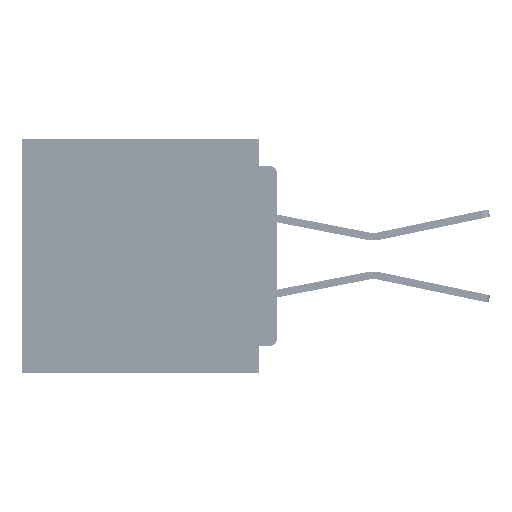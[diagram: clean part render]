
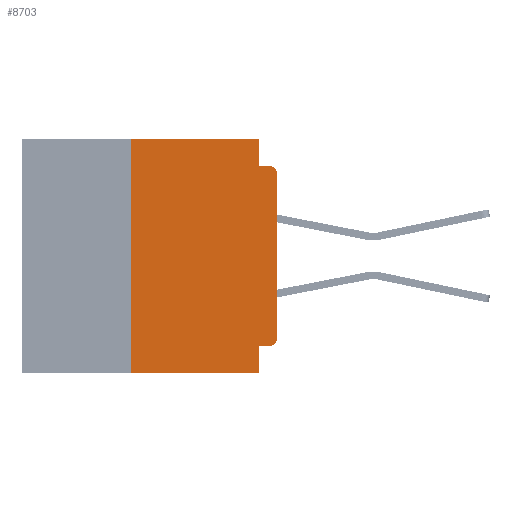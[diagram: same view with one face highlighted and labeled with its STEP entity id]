
A CAD part, left-side view. The second image highlights one B-rep face of the part: STEP entity #8703.
In plain terms, the highlighted planar face has unit normal (-1, 0, 0).
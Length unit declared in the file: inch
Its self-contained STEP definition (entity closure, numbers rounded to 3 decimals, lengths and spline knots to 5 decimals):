
#1179 = ORIENTED_EDGE ( 'NONE', *, *, #52710, .T. ) ;
#2013 = VERTEX_POINT ( 'NONE', #58981 ) ;
#2513 = VECTOR ( 'NONE', #21681, 39.37008 ) ;
#3818 = DIRECTION ( 'NONE',  ( 0., -1., 0. ) ) ;
#4397 = EDGE_CURVE ( 'NONE', #4600, #26843, #53776, .T. ) ;
#4600 = VERTEX_POINT ( 'NONE', #53090 ) ;
#5264 = CARTESIAN_POINT ( 'NONE',  ( 0., 0.437, 0. ) ) ;
#6177 = AXIS2_PLACEMENT_3D ( 'NONE', #39519, #9845, #44536 ) ;
#7293 = LINE ( 'NONE', #63504, #32089 ) ;
#7843 = EDGE_CURVE ( 'NONE', #55720, #57735, #31541, .T. ) ;
#8025 = CARTESIAN_POINT ( 'NONE',  ( 0., 0.031, 0. ) ) ;
#8219 = CARTESIAN_POINT ( 'NONE',  ( 0., 0.031, -0.4 ) ) ;
#8703 = ADVANCED_FACE ( 'NONE', ( #63314 ), #39957, .F. ) ;
#9010 = ORIENTED_EDGE ( 'NONE', *, *, #55479, .T. ) ;
#9325 = ORIENTED_EDGE ( 'NONE', *, *, #24164, .F. ) ;
#9845 = DIRECTION ( 'NONE',  ( -1., 0., 0. ) ) ;
#10053 = CARTESIAN_POINT ( 'NONE',  ( 0., 0.031, -0.4 ) ) ;
#12025 = ORIENTED_EDGE ( 'NONE', *, *, #29347, .T. ) ;
#13001 = DIRECTION ( 'NONE',  ( -1., 0., 0. ) ) ;
#14952 = CARTESIAN_POINT ( 'NONE',  ( 0., 0.437, -0.4 ) ) ;
#18389 = VECTOR ( 'NONE', #28321, 39.37008 ) ;
#18434 = CARTESIAN_POINT ( 'NONE',  ( 0., 0.25, -0.4 ) ) ;
#18601 = AXIS2_PLACEMENT_3D ( 'NONE', #42706, #13001, #47699 ) ;
#19692 = CARTESIAN_POINT ( 'NONE',  ( 0., 0., -0.34 ) ) ;
#21681 = DIRECTION ( 'NONE',  ( 0., 1., 0. ) ) ;
#23253 = VECTOR ( 'NONE', #60060, 39.37008 ) ;
#23881 = DIRECTION ( 'NONE',  ( 0., 0., -1. ) ) ;
#24164 = EDGE_CURVE ( 'NONE', #2013, #37895, #37993, .T. ) ;
#25200 = DIRECTION ( 'NONE',  ( 1., 0., 0. ) ) ;
#25498 = ORIENTED_EDGE ( 'NONE', *, *, #46148, .T. ) ;
#26021 = LINE ( 'NONE', #8219, #34549 ) ;
#26295 = EDGE_CURVE ( 'NONE', #26843, #31325, #26021, .T. ) ;
#26628 = ORIENTED_EDGE ( 'NONE', *, *, #59105, .F. ) ;
#26843 = VERTEX_POINT ( 'NONE', #42211 ) ;
#27868 = AXIS2_PLACEMENT_3D ( 'NONE', #5264, #25200, #59905 ) ;
#28321 = DIRECTION ( 'NONE',  ( 0., 0., 1. ) ) ;
#29347 = EDGE_CURVE ( 'NONE', #30622, #50250, #49211, .T. ) ;
#29992 = VECTOR ( 'NONE', #3818, 39.37008 ) ;
#30622 = VERTEX_POINT ( 'NONE', #19692 ) ;
#31325 = VERTEX_POINT ( 'NONE', #10053 ) ;
#31541 = LINE ( 'NONE', #63206, #29992 ) ;
#32089 = VECTOR ( 'NONE', #23881, 39.37008 ) ;
#34108 = VECTOR ( 'NONE', #49672, 39.37008 ) ;
#34346 = DIRECTION ( 'NONE',  ( 0., 0., 1. ) ) ;
#34549 = VECTOR ( 'NONE', #37917, 39.37008 ) ;
#34897 = CARTESIAN_POINT ( 'NONE',  ( 0., 0.015, -0.045 ) ) ;
#35275 = CIRCLE ( 'NONE', #18601, 0.015 ) ;
#35688 = ORIENTED_EDGE ( 'NONE', *, *, #4397, .F. ) ;
#35989 = VECTOR ( 'NONE', #34346, 39.37008 ) ;
#36481 = CARTESIAN_POINT ( 'NONE',  ( 0., 0.031, -0.045 ) ) ;
#37278 = CARTESIAN_POINT ( 'NONE',  ( 0., 0.25, -0.4 ) ) ;
#37562 = CARTESIAN_POINT ( 'NONE',  ( 0., 0., -0.06 ) ) ;
#37743 = EDGE_LOOP ( 'NONE', ( #12025, #1179, #56136, #26628, #9325, #55139, #25498, #40042, #35688, #9010 ) ) ;
#37895 = VERTEX_POINT ( 'NONE', #8025 ) ;
#37917 = DIRECTION ( 'NONE',  ( 0., 0., -1. ) ) ;
#37993 = LINE ( 'NONE', #55073, #23253 ) ;
#39519 = CARTESIAN_POINT ( 'NONE',  ( 0., 0.015, -0.34 ) ) ;
#39957 = PLANE ( 'NONE',  #27868 ) ;
#40042 = ORIENTED_EDGE ( 'NONE', *, *, #26295, .F. ) ;
#42211 = CARTESIAN_POINT ( 'NONE',  ( 0., 0.031, -0.355 ) ) ;
#42706 = CARTESIAN_POINT ( 'NONE',  ( 0., 0.015, -0.06 ) ) ;
#44536 = DIRECTION ( 'NONE',  ( 0., 0., -1. ) ) ;
#44723 = EDGE_CURVE ( 'NONE', #52684, #2013, #57917, .T. ) ;
#46148 = EDGE_CURVE ( 'NONE', #52684, #31325, #47368, .T. ) ;
#47368 = LINE ( 'NONE', #14952, #34108 ) ;
#47699 = DIRECTION ( 'NONE',  ( 0., 0., -1. ) ) ;
#49211 = LINE ( 'NONE', #54116, #35989 ) ;
#49672 = DIRECTION ( 'NONE',  ( 0., -1., 0. ) ) ;
#50250 = VERTEX_POINT ( 'NONE', #37562 ) ;
#52684 = VERTEX_POINT ( 'NONE', #37278 ) ;
#52710 = EDGE_CURVE ( 'NONE', #50250, #57735, #35275, .T. ) ;
#53090 = CARTESIAN_POINT ( 'NONE',  ( 0., 0.015, -0.355 ) ) ;
#53776 = LINE ( 'NONE', #56333, #2513 ) ;
#54116 = CARTESIAN_POINT ( 'NONE',  ( 0., 0., 0. ) ) ;
#54414 = CIRCLE ( 'NONE', #6177, 0.015 ) ;
#55073 = CARTESIAN_POINT ( 'NONE',  ( 0., 0.437, 0. ) ) ;
#55139 = ORIENTED_EDGE ( 'NONE', *, *, #44723, .F. ) ;
#55479 = EDGE_CURVE ( 'NONE', #4600, #30622, #54414, .T. ) ;
#55720 = VERTEX_POINT ( 'NONE', #36481 ) ;
#56136 = ORIENTED_EDGE ( 'NONE', *, *, #7843, .F. ) ;
#56333 = CARTESIAN_POINT ( 'NONE',  ( 0., 0., -0.355 ) ) ;
#57735 = VERTEX_POINT ( 'NONE', #34897 ) ;
#57917 = LINE ( 'NONE', #18434, #18389 ) ;
#58981 = CARTESIAN_POINT ( 'NONE',  ( 0., 0.25, 0. ) ) ;
#59105 = EDGE_CURVE ( 'NONE', #37895, #55720, #7293, .T. ) ;
#59905 = DIRECTION ( 'NONE',  ( 0., 0., -1. ) ) ;
#60060 = DIRECTION ( 'NONE',  ( 0., -1., 0. ) ) ;
#63206 = CARTESIAN_POINT ( 'NONE',  ( 0., 0., -0.045 ) ) ;
#63314 = FACE_OUTER_BOUND ( 'NONE', #37743, .T. ) ;
#63504 = CARTESIAN_POINT ( 'NONE',  ( 0., 0.031, 0. ) ) ;
